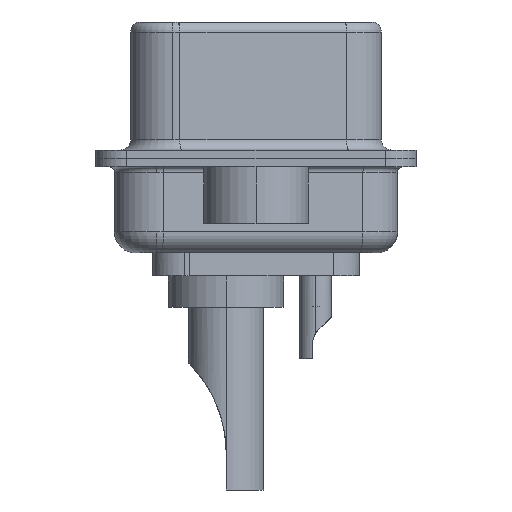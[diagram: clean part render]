
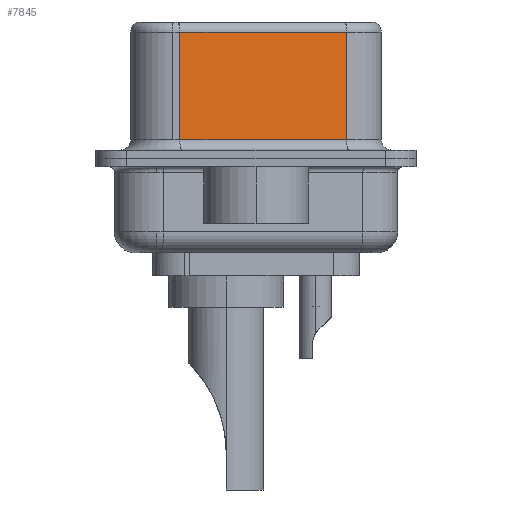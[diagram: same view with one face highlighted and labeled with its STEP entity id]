
A CAD part, left-side view. The second image highlights one B-rep face of the part: STEP entity #7845.
In plain terms, the highlighted planar face has unit normal (-0.985, -0.174, 0).
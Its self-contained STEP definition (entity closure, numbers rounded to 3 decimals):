
#708 = VECTOR ( 'NONE', #13576, 1000. ) ;
#1375 = VERTEX_POINT ( 'NONE', #14063 ) ;
#2035 = PLANE ( 'NONE',  #10188 ) ;
#3332 = DIRECTION ( 'NONE',  ( -0.174, 0.985, 0. ) ) ;
#3492 = LINE ( 'NONE', #7626, #15821 ) ;
#3518 = EDGE_CURVE ( 'NONE', #1375, #16276, #9687, .T. ) ;
#5086 = ORIENTED_EDGE ( 'NONE', *, *, #3518, .T. ) ;
#5158 = CARTESIAN_POINT ( 'NONE',  ( 5.132, -4.322, 6.02 ) ) ;
#5564 = CARTESIAN_POINT ( 'NONE',  ( 5.132, -4.322, 0.9 ) ) ;
#5807 = FACE_OUTER_BOUND ( 'NONE', #6884, .T. ) ;
#5843 = DIRECTION ( 'NONE',  ( -0.174, 0.985, 0. ) ) ;
#6010 = DIRECTION ( 'NONE',  ( 0.985, 0.174, 0. ) ) ;
#6076 = CARTESIAN_POINT ( 'NONE',  ( 5.132, -4.322, 6.52 ) ) ;
#6222 = EDGE_CURVE ( 'NONE', #19554, #15785, #3492, .T. ) ;
#6884 = EDGE_LOOP ( 'NONE', ( #20000, #9787, #15243, #5086 ) ) ;
#7626 = CARTESIAN_POINT ( 'NONE',  ( 5.132, -4.322, 6.02 ) ) ;
#7845 = ADVANCED_FACE ( 'NONE', ( #5807 ), #2035, .F. ) ;
#9687 = LINE ( 'NONE', #13428, #708 ) ;
#9787 = ORIENTED_EDGE ( 'NONE', *, *, #6222, .T. ) ;
#10140 = LINE ( 'NONE', #18970, #14027 ) ;
#10188 = AXIS2_PLACEMENT_3D ( 'NONE', #6076, #6010, #5843 ) ;
#10782 = EDGE_CURVE ( 'NONE', #15785, #1375, #10140, .T. ) ;
#11596 = VECTOR ( 'NONE', #13079, 1000. ) ;
#13079 = DIRECTION ( 'NONE',  ( 0., 0., -1. ) ) ;
#13428 = CARTESIAN_POINT ( 'NONE',  ( 5.132, -4.322, 0.9 ) ) ;
#13576 = DIRECTION ( 'NONE',  ( 0.174, -0.985, 0. ) ) ;
#13850 = DIRECTION ( 'NONE',  ( 0., 0., -1. ) ) ;
#14027 = VECTOR ( 'NONE', #13850, 1000. ) ;
#14063 = CARTESIAN_POINT ( 'NONE',  ( 3.73, 3.628, 0.9 ) ) ;
#14800 = CARTESIAN_POINT ( 'NONE',  ( 5.132, -4.322, 6.52 ) ) ;
#15243 = ORIENTED_EDGE ( 'NONE', *, *, #10782, .T. ) ;
#15785 = VERTEX_POINT ( 'NONE', #19664 ) ;
#15821 = VECTOR ( 'NONE', #3332, 1000. ) ;
#15886 = EDGE_CURVE ( 'NONE', #19554, #16276, #16100, .T. ) ;
#16100 = LINE ( 'NONE', #14800, #11596 ) ;
#16276 = VERTEX_POINT ( 'NONE', #5564 ) ;
#18970 = CARTESIAN_POINT ( 'NONE',  ( 3.73, 3.628, 6.52 ) ) ;
#19554 = VERTEX_POINT ( 'NONE', #5158 ) ;
#19664 = CARTESIAN_POINT ( 'NONE',  ( 3.73, 3.628, 6.02 ) ) ;
#20000 = ORIENTED_EDGE ( 'NONE', *, *, #15886, .F. ) ;
